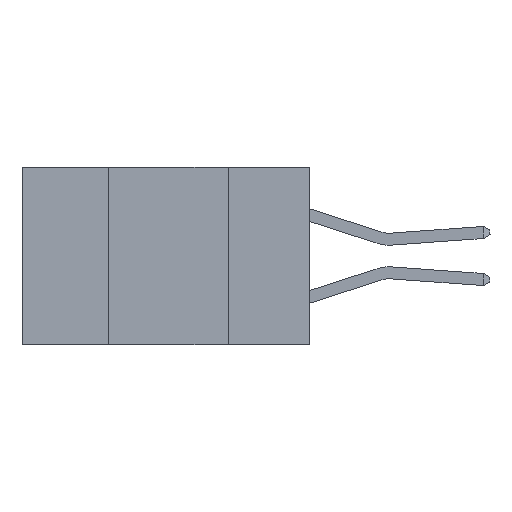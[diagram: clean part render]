
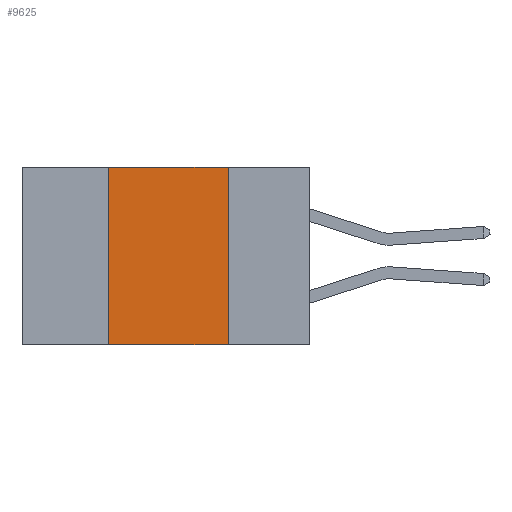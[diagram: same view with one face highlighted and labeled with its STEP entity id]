
A CAD part, left-side view. The second image highlights one B-rep face of the part: STEP entity #9625.
In plain terms, the highlighted planar face has unit normal (-1, 0, 0).
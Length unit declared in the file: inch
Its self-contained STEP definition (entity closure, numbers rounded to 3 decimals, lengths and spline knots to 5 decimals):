
#150 = ORIENTED_EDGE ( 'NONE', *, *, #9885, .T. ) ;
#365 = VERTEX_POINT ( 'NONE', #19204 ) ;
#369 = EDGE_CURVE ( 'NONE', #12604, #21095, #12830, .T. ) ;
#409 = LINE ( 'NONE', #19837, #24706 ) ;
#1467 = DIRECTION ( 'NONE',  ( 0., -1., 0. ) ) ;
#1850 = VECTOR ( 'NONE', #13836, 39.37008 ) ;
#2677 = CARTESIAN_POINT ( 'NONE',  ( 0., 0.42, -0.37 ) ) ;
#3522 = LINE ( 'NONE', #7518, #22786 ) ;
#4204 = CARTESIAN_POINT ( 'NONE',  ( 0., 0.6, 0. ) ) ;
#5937 = CARTESIAN_POINT ( 'NONE',  ( 0., 0.42, -0.37 ) ) ;
#6333 = ORIENTED_EDGE ( 'NONE', *, *, #19543, .F. ) ;
#6763 = DIRECTION ( 'NONE',  ( 0., -1., 0. ) ) ;
#6893 = DIRECTION ( 'NONE',  ( 0., 0., -1. ) ) ;
#7177 = CARTESIAN_POINT ( 'NONE',  ( 0., 0.42, 0. ) ) ;
#7485 = LINE ( 'NONE', #5937, #1850 ) ;
#7518 = CARTESIAN_POINT ( 'NONE',  ( 0., 0.6, -0.37 ) ) ;
#8072 = FACE_OUTER_BOUND ( 'NONE', #13154, .T. ) ;
#9562 = VECTOR ( 'NONE', #6763, 39.37008 ) ;
#9625 = ADVANCED_FACE ( 'NONE', ( #8072 ), #15937, .F. ) ;
#9885 = EDGE_CURVE ( 'NONE', #13007, #365, #3522, .T. ) ;
#11332 = AXIS2_PLACEMENT_3D ( 'NONE', #4204, #12079, #6893 ) ;
#11608 = EDGE_CURVE ( 'NONE', #13007, #12604, #7485, .T. ) ;
#11761 = ORIENTED_EDGE ( 'NONE', *, *, #369, .F. ) ;
#12079 = DIRECTION ( 'NONE',  ( 1., 0., 0. ) ) ;
#12604 = VERTEX_POINT ( 'NONE', #7177 ) ;
#12830 = LINE ( 'NONE', #13315, #9562 ) ;
#13007 = VERTEX_POINT ( 'NONE', #2677 ) ;
#13154 = EDGE_LOOP ( 'NONE', ( #6333, #11761, #16995, #150 ) ) ;
#13315 = CARTESIAN_POINT ( 'NONE',  ( 0., 0.6, 0. ) ) ;
#13836 = DIRECTION ( 'NONE',  ( 0., 0., 1. ) ) ;
#15937 = PLANE ( 'NONE',  #11332 ) ;
#16995 = ORIENTED_EDGE ( 'NONE', *, *, #11608, .F. ) ;
#19204 = CARTESIAN_POINT ( 'NONE',  ( 0., 0.17, -0.37 ) ) ;
#19543 = EDGE_CURVE ( 'NONE', #21095, #365, #409, .T. ) ;
#19837 = CARTESIAN_POINT ( 'NONE',  ( 0., 0.17, -0.37 ) ) ;
#21095 = VERTEX_POINT ( 'NONE', #22175 ) ;
#22175 = CARTESIAN_POINT ( 'NONE',  ( 0., 0.17, 0. ) ) ;
#22786 = VECTOR ( 'NONE', #1467, 39.37008 ) ;
#24182 = DIRECTION ( 'NONE',  ( 0., 0., -1. ) ) ;
#24706 = VECTOR ( 'NONE', #24182, 39.37008 ) ;
